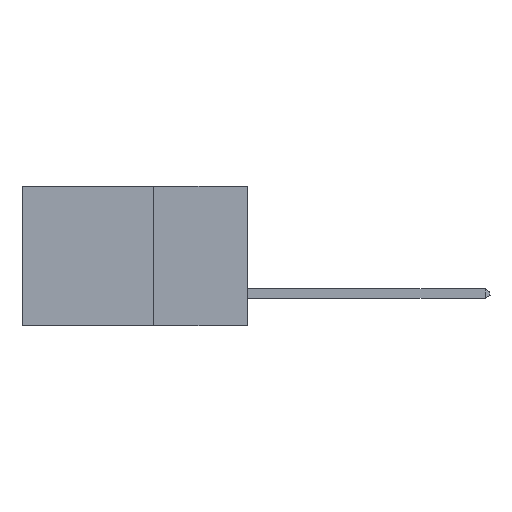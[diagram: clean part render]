
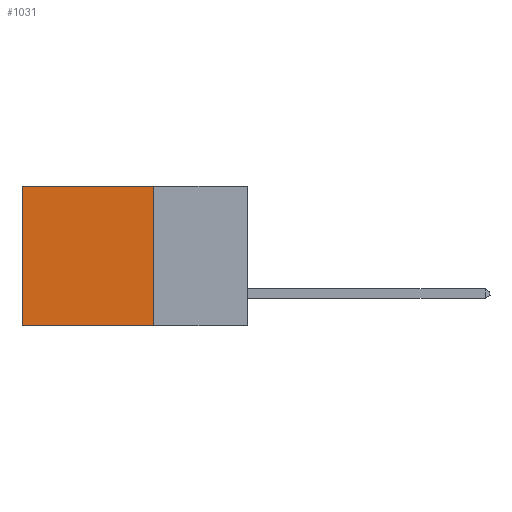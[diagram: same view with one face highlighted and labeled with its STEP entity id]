
A CAD part, left-side view. The second image highlights one B-rep face of the part: STEP entity #1031.
In plain terms, the highlighted planar face has unit normal (-1, 0, 0).
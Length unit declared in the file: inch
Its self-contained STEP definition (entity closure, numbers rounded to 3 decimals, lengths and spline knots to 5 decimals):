
#232 = VECTOR ( 'NONE', #11354, 39.37008 ) ;
#519 = LINE ( 'NONE', #6295, #13175 ) ;
#1031 = ADVANCED_FACE ( 'NONE', ( #13518 ), #6701, .F. ) ;
#1143 = ORIENTED_EDGE ( 'NONE', *, *, #16884, .T. ) ;
#1225 = CARTESIAN_POINT ( 'NONE',  ( 0.298, 0.25, 0. ) ) ;
#1815 = CARTESIAN_POINT ( 'NONE',  ( 0.298, 0.6, -0.37 ) ) ;
#1942 = LINE ( 'NONE', #11894, #15417 ) ;
#1947 = ORIENTED_EDGE ( 'NONE', *, *, #8250, .T. ) ;
#3111 = CARTESIAN_POINT ( 'NONE',  ( 0.298, 0.25, -0.37 ) ) ;
#3155 = VERTEX_POINT ( 'NONE', #3111 ) ;
#3638 = VERTEX_POINT ( 'NONE', #4709 ) ;
#4472 = EDGE_CURVE ( 'NONE', #3155, #15483, #519, .T. ) ;
#4692 = CARTESIAN_POINT ( 'NONE',  ( 0.298, 0.6, 0. ) ) ;
#4709 = CARTESIAN_POINT ( 'NONE',  ( 0.298, 0.25, 0. ) ) ;
#5017 = DIRECTION ( 'NONE',  ( 0., 1., 0. ) ) ;
#6295 = CARTESIAN_POINT ( 'NONE',  ( 0.298, 0.25, -0.37 ) ) ;
#6701 = PLANE ( 'NONE',  #11462 ) ;
#6813 = DIRECTION ( 'NONE',  ( 1., 0., 0. ) ) ;
#7224 = VERTEX_POINT ( 'NONE', #4692 ) ;
#7742 = LINE ( 'NONE', #8660, #232 ) ;
#8250 = EDGE_CURVE ( 'NONE', #3638, #7224, #7742, .T. ) ;
#8660 = CARTESIAN_POINT ( 'NONE',  ( 0.298, 0.25, 0. ) ) ;
#9584 = VECTOR ( 'NONE', #14839, 39.37008 ) ;
#10707 = DIRECTION ( 'NONE',  ( 0., 0., -1. ) ) ;
#10795 = DIRECTION ( 'NONE',  ( 0., 0., -1. ) ) ;
#11098 = ORIENTED_EDGE ( 'NONE', *, *, #11638, .F. ) ;
#11354 = DIRECTION ( 'NONE',  ( 0., 1., 0. ) ) ;
#11462 = AXIS2_PLACEMENT_3D ( 'NONE', #1225, #6813, #10795 ) ;
#11600 = EDGE_LOOP ( 'NONE', ( #1143, #13357, #11098, #1947 ) ) ;
#11638 = EDGE_CURVE ( 'NONE', #3638, #3155, #14938, .T. ) ;
#11894 = CARTESIAN_POINT ( 'NONE',  ( 0.298, 0.6, 0. ) ) ;
#13175 = VECTOR ( 'NONE', #5017, 39.37008 ) ;
#13357 = ORIENTED_EDGE ( 'NONE', *, *, #4472, .F. ) ;
#13518 = FACE_OUTER_BOUND ( 'NONE', #11600, .T. ) ;
#13718 = CARTESIAN_POINT ( 'NONE',  ( 0.298, 0.25, 0. ) ) ;
#14839 = DIRECTION ( 'NONE',  ( 0., 0., -1. ) ) ;
#14938 = LINE ( 'NONE', #13718, #9584 ) ;
#15417 = VECTOR ( 'NONE', #10707, 39.37008 ) ;
#15483 = VERTEX_POINT ( 'NONE', #1815 ) ;
#16884 = EDGE_CURVE ( 'NONE', #7224, #15483, #1942, .T. ) ;
